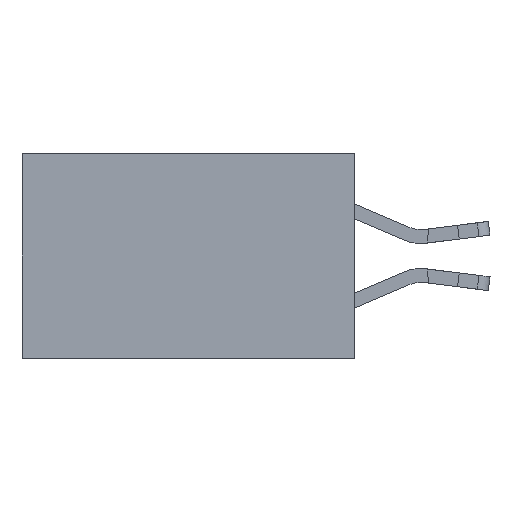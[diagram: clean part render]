
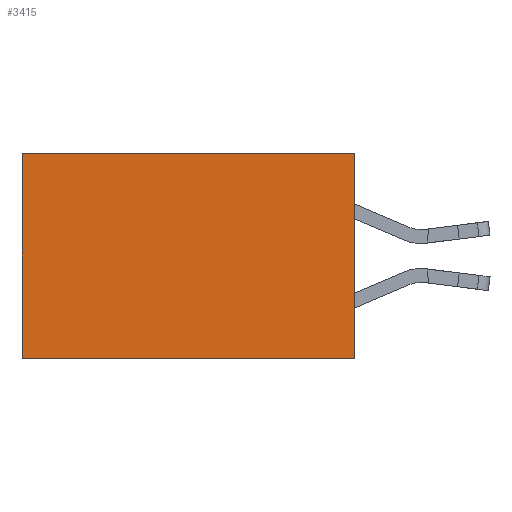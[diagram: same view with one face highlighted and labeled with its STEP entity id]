
A CAD part, left-side view. The second image highlights one B-rep face of the part: STEP entity #3415.
In plain terms, the highlighted planar face has unit normal (-1, 0, 0).
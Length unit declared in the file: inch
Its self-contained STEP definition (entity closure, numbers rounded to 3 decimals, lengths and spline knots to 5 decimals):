
#287 = DIRECTION ( 'NONE',  ( 0., 0., -1. ) ) ;
#1723 = VECTOR ( 'NONE', #14324, 39.37008 ) ;
#2437 = CARTESIAN_POINT ( 'NONE',  ( 0.298, 0.6, 0. ) ) ;
#2484 = CARTESIAN_POINT ( 'NONE',  ( 0.298, 0., 0. ) ) ;
#3415 = ADVANCED_FACE ( 'NONE', ( #3600 ), #4644, .F. ) ;
#3600 = FACE_OUTER_BOUND ( 'NONE', #15181, .T. ) ;
#3729 = CARTESIAN_POINT ( 'NONE',  ( 0.298, 0., 0. ) ) ;
#4347 = VERTEX_POINT ( 'NONE', #2437 ) ;
#4644 = PLANE ( 'NONE',  #12691 ) ;
#4721 = ORIENTED_EDGE ( 'NONE', *, *, #14689, .F. ) ;
#5399 = CARTESIAN_POINT ( 'NONE',  ( 0.298, 0., -0.37 ) ) ;
#6110 = EDGE_CURVE ( 'NONE', #11202, #4347, #9788, .T. ) ;
#7309 = VERTEX_POINT ( 'NONE', #5399 ) ;
#7372 = LINE ( 'NONE', #2484, #12008 ) ;
#7521 = DIRECTION ( 'NONE',  ( 0., 1., 0. ) ) ;
#7823 = CARTESIAN_POINT ( 'NONE',  ( 0.298, 0.6, 0. ) ) ;
#7963 = CARTESIAN_POINT ( 'NONE',  ( 0.298, 0., 0. ) ) ;
#8155 = ORIENTED_EDGE ( 'NONE', *, *, #10976, .T. ) ;
#8437 = LINE ( 'NONE', #7823, #9928 ) ;
#8492 = VERTEX_POINT ( 'NONE', #14224 ) ;
#8686 = VECTOR ( 'NONE', #7521, 39.37008 ) ;
#8813 = CARTESIAN_POINT ( 'NONE',  ( 0.298, 0., -0.37 ) ) ;
#9040 = LINE ( 'NONE', #8813, #8686 ) ;
#9788 = LINE ( 'NONE', #10771, #1723 ) ;
#9829 = ORIENTED_EDGE ( 'NONE', *, *, #14914, .F. ) ;
#9928 = VECTOR ( 'NONE', #13752, 39.37008 ) ;
#10501 = DIRECTION ( 'NONE',  ( 1., 0., 0. ) ) ;
#10771 = CARTESIAN_POINT ( 'NONE',  ( 0.298, 0., 0. ) ) ;
#10976 = EDGE_CURVE ( 'NONE', #4347, #8492, #8437, .T. ) ;
#11202 = VERTEX_POINT ( 'NONE', #3729 ) ;
#11659 = ORIENTED_EDGE ( 'NONE', *, *, #6110, .T. ) ;
#12008 = VECTOR ( 'NONE', #287, 39.37008 ) ;
#12691 = AXIS2_PLACEMENT_3D ( 'NONE', #7963, #10501, #13935 ) ;
#13752 = DIRECTION ( 'NONE',  ( 0., 0., -1. ) ) ;
#13935 = DIRECTION ( 'NONE',  ( 0., 0., -1. ) ) ;
#14224 = CARTESIAN_POINT ( 'NONE',  ( 0.298, 0.6, -0.37 ) ) ;
#14324 = DIRECTION ( 'NONE',  ( 0., 1., 0. ) ) ;
#14689 = EDGE_CURVE ( 'NONE', #7309, #8492, #9040, .T. ) ;
#14914 = EDGE_CURVE ( 'NONE', #11202, #7309, #7372, .T. ) ;
#15181 = EDGE_LOOP ( 'NONE', ( #8155, #4721, #9829, #11659 ) ) ;
